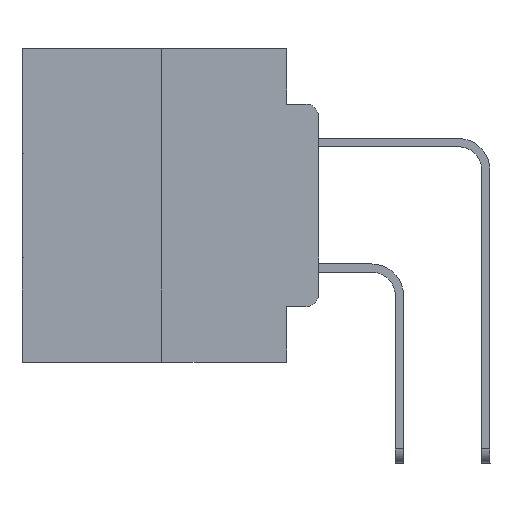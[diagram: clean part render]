
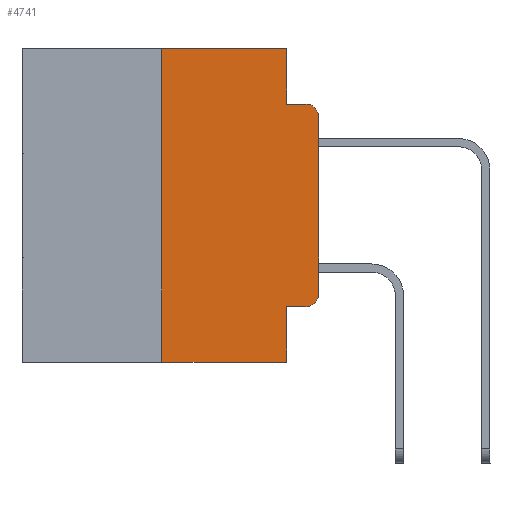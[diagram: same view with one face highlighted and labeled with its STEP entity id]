
A CAD part, left-side view. The second image highlights one B-rep face of the part: STEP entity #4741.
In plain terms, the highlighted planar face has unit normal (-1, 0, 0).
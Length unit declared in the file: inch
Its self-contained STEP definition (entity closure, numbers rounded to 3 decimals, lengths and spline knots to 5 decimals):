
#35 = VERTEX_POINT ( 'NONE', #3444 ) ;
#513 = ORIENTED_EDGE ( 'NONE', *, *, #2059, .T. ) ;
#788 = ORIENTED_EDGE ( 'NONE', *, *, #26304, .T. ) ;
#1408 = LINE ( 'NONE', #5845, #25782 ) ;
#1457 = CARTESIAN_POINT ( 'NONE',  ( 0., 0.051, 0. ) ) ;
#1537 = ORIENTED_EDGE ( 'NONE', *, *, #2844, .T. ) ;
#1550 = LINE ( 'NONE', #12200, #13605 ) ;
#1820 = CARTESIAN_POINT ( 'NONE',  ( 0., 0.02, -0.1085 ) ) ;
#1867 = EDGE_CURVE ( 'NONE', #10960, #20689, #14290, .T. ) ;
#2059 = EDGE_CURVE ( 'NONE', #27005, #35, #13910, .T. ) ;
#2385 = CARTESIAN_POINT ( 'NONE',  ( 0., 0.473, 0. ) ) ;
#2844 = EDGE_CURVE ( 'NONE', #26113, #23828, #25813, .T. ) ;
#2928 = VECTOR ( 'NONE', #29484, 39.37008 ) ;
#3116 = VERTEX_POINT ( 'NONE', #15246 ) ;
#3285 = EDGE_CURVE ( 'NONE', #3116, #10151, #1408, .T. ) ;
#3444 = CARTESIAN_POINT ( 'NONE',  ( 0., 0., -0.1085 ) ) ;
#3488 = VERTEX_POINT ( 'NONE', #3920 ) ;
#3920 = CARTESIAN_POINT ( 'NONE',  ( 0., 0.02, -0.0885 ) ) ;
#4312 = DIRECTION ( 'NONE',  ( 0., 0., -1. ) ) ;
#4741 = ADVANCED_FACE ( 'NONE', ( #5982 ), #28266, .F. ) ;
#5845 = CARTESIAN_POINT ( 'NONE',  ( 0., 0.051, -0.4115 ) ) ;
#5982 = FACE_OUTER_BOUND ( 'NONE', #9010, .T. ) ;
#6295 = DIRECTION ( 'NONE',  ( 0., -1., 0. ) ) ;
#7303 = CARTESIAN_POINT ( 'NONE',  ( 0., 0.25, 0. ) ) ;
#9010 = EDGE_LOOP ( 'NONE', ( #513, #788, #24496, #11068, #24224, #22109, #1537, #13673, #23145, #24105 ) ) ;
#9343 = CARTESIAN_POINT ( 'NONE',  ( 0., 0., -0.3915 ) ) ;
#9360 = AXIS2_PLACEMENT_3D ( 'NONE', #24074, #10153, #26337 ) ;
#9742 = DIRECTION ( 'NONE',  ( 0., 0., 1. ) ) ;
#9803 = EDGE_CURVE ( 'NONE', #3116, #23828, #15642, .T. ) ;
#10151 = VERTEX_POINT ( 'NONE', #19238 ) ;
#10153 = DIRECTION ( 'NONE',  ( -1., 0., 0. ) ) ;
#10449 = CIRCLE ( 'NONE', #9360, 0.02 ) ;
#10806 = EDGE_CURVE ( 'NONE', #20689, #22228, #18844, .T. ) ;
#10950 = VECTOR ( 'NONE', #9742, 39.37008 ) ;
#10960 = VERTEX_POINT ( 'NONE', #29033 ) ;
#11068 = ORIENTED_EDGE ( 'NONE', *, *, #10806, .F. ) ;
#12200 = CARTESIAN_POINT ( 'NONE',  ( 0., 0.051, -0.0885 ) ) ;
#13605 = VECTOR ( 'NONE', #14551, 39.37008 ) ;
#13673 = ORIENTED_EDGE ( 'NONE', *, *, #9803, .F. ) ;
#13693 = DIRECTION ( 'NONE',  ( 0., 0., -1. ) ) ;
#13910 = LINE ( 'NONE', #27902, #25512 ) ;
#14086 = AXIS2_PLACEMENT_3D ( 'NONE', #17496, #16904, #13693 ) ;
#14290 = LINE ( 'NONE', #2385, #25176 ) ;
#14551 = DIRECTION ( 'NONE',  ( 0., -1., 0. ) ) ;
#15246 = CARTESIAN_POINT ( 'NONE',  ( 0., 0.051, -0.4115 ) ) ;
#15642 = LINE ( 'NONE', #1457, #2928 ) ;
#16748 = DIRECTION ( 'NONE',  ( 0., 0., 1. ) ) ;
#16904 = DIRECTION ( 'NONE',  ( 1., 0., 0. ) ) ;
#17086 = EDGE_CURVE ( 'NONE', #22228, #3488, #1550, .T. ) ;
#17496 = CARTESIAN_POINT ( 'NONE',  ( 0., 0.473, 0. ) ) ;
#18498 = DIRECTION ( 'NONE',  ( -1., 0., 0. ) ) ;
#18844 = LINE ( 'NONE', #28462, #30217 ) ;
#19238 = CARTESIAN_POINT ( 'NONE',  ( 0., 0.02, -0.4115 ) ) ;
#19407 = DIRECTION ( 'NONE',  ( 0., 0., -1. ) ) ;
#19429 = CARTESIAN_POINT ( 'NONE',  ( 0., 0.051, 0. ) ) ;
#20024 = CARTESIAN_POINT ( 'NONE',  ( 0., 0.25, -0.5 ) ) ;
#20424 = VECTOR ( 'NONE', #22472, 39.37008 ) ;
#20689 = VERTEX_POINT ( 'NONE', #19429 ) ;
#21295 = AXIS2_PLACEMENT_3D ( 'NONE', #1820, #18498, #4312 ) ;
#22109 = ORIENTED_EDGE ( 'NONE', *, *, #29837, .F. ) ;
#22228 = VERTEX_POINT ( 'NONE', #27139 ) ;
#22472 = DIRECTION ( 'NONE',  ( 0., -1., 0. ) ) ;
#22478 = CARTESIAN_POINT ( 'NONE',  ( 0., 0.473, -0.5 ) ) ;
#22794 = CIRCLE ( 'NONE', #21295, 0.02 ) ;
#23145 = ORIENTED_EDGE ( 'NONE', *, *, #3285, .T. ) ;
#23310 = DIRECTION ( 'NONE',  ( 0., -1., 0. ) ) ;
#23826 = CARTESIAN_POINT ( 'NONE',  ( 0., 0.051, -0.5 ) ) ;
#23828 = VERTEX_POINT ( 'NONE', #23826 ) ;
#24074 = CARTESIAN_POINT ( 'NONE',  ( 0., 0.02, -0.3915 ) ) ;
#24105 = ORIENTED_EDGE ( 'NONE', *, *, #25929, .T. ) ;
#24224 = ORIENTED_EDGE ( 'NONE', *, *, #1867, .F. ) ;
#24496 = ORIENTED_EDGE ( 'NONE', *, *, #17086, .F. ) ;
#25176 = VECTOR ( 'NONE', #23310, 39.37008 ) ;
#25512 = VECTOR ( 'NONE', #16748, 39.37008 ) ;
#25782 = VECTOR ( 'NONE', #6295, 39.37008 ) ;
#25813 = LINE ( 'NONE', #22478, #20424 ) ;
#25929 = EDGE_CURVE ( 'NONE', #10151, #27005, #10449, .T. ) ;
#26113 = VERTEX_POINT ( 'NONE', #20024 ) ;
#26304 = EDGE_CURVE ( 'NONE', #35, #3488, #22794, .T. ) ;
#26337 = DIRECTION ( 'NONE',  ( 0., 0., -1. ) ) ;
#27005 = VERTEX_POINT ( 'NONE', #9343 ) ;
#27139 = CARTESIAN_POINT ( 'NONE',  ( 0., 0.051, -0.0885 ) ) ;
#27902 = CARTESIAN_POINT ( 'NONE',  ( 0., 0., 0. ) ) ;
#28266 = PLANE ( 'NONE',  #14086 ) ;
#28462 = CARTESIAN_POINT ( 'NONE',  ( 0., 0.051, 0. ) ) ;
#29033 = CARTESIAN_POINT ( 'NONE',  ( 0., 0.25, 0. ) ) ;
#29281 = LINE ( 'NONE', #7303, #10950 ) ;
#29484 = DIRECTION ( 'NONE',  ( 0., 0., -1. ) ) ;
#29837 = EDGE_CURVE ( 'NONE', #26113, #10960, #29281, .T. ) ;
#30217 = VECTOR ( 'NONE', #19407, 39.37008 ) ;
